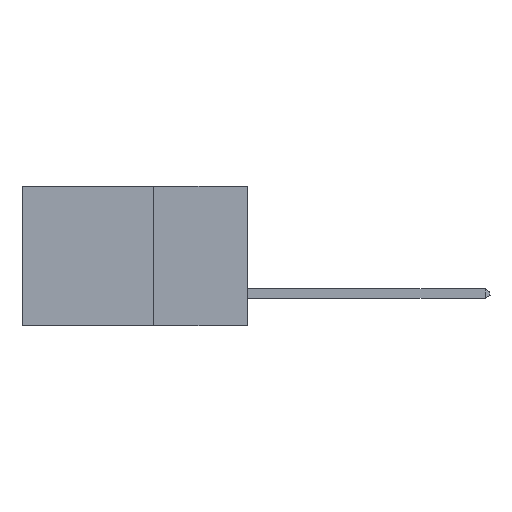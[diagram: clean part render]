
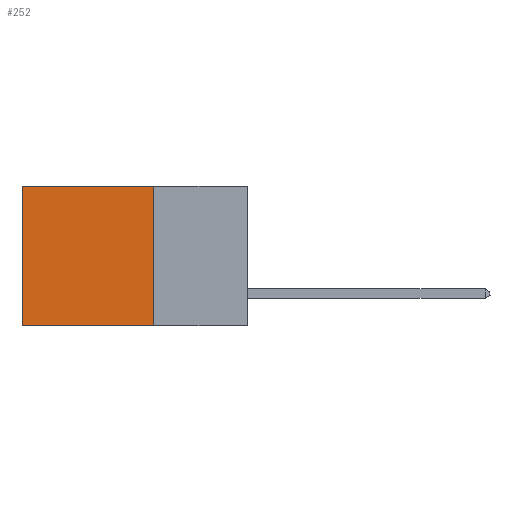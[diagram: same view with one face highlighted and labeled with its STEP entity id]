
A CAD part, left-side view. The second image highlights one B-rep face of the part: STEP entity #252.
In plain terms, the highlighted planar face has unit normal (-1, 0, 0).
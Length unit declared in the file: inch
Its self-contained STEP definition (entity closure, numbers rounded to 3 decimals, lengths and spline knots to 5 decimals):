
#252 = ADVANCED_FACE ( 'NONE', ( #9897 ), #10435, .F. ) ;
#400 = DIRECTION ( 'NONE',  ( 0., 1., 0. ) ) ;
#653 = VECTOR ( 'NONE', #4759, 39.37008 ) ;
#1250 = CARTESIAN_POINT ( 'NONE',  ( 0.298, 0.6, 0. ) ) ;
#1573 = CARTESIAN_POINT ( 'NONE',  ( 0.298, 0.6, 0. ) ) ;
#1584 = LINE ( 'NONE', #4831, #7233 ) ;
#1799 = DIRECTION ( 'NONE',  ( 0., 1., 0. ) ) ;
#3656 = CARTESIAN_POINT ( 'NONE',  ( 0.298, 0.25, 0. ) ) ;
#3745 = VERTEX_POINT ( 'NONE', #3656 ) ;
#3851 = EDGE_CURVE ( 'NONE', #3745, #8096, #1584, .T. ) ;
#4073 = LINE ( 'NONE', #1573, #653 ) ;
#4759 = DIRECTION ( 'NONE',  ( 0., 0., -1. ) ) ;
#4831 = CARTESIAN_POINT ( 'NONE',  ( 0.298, 0.25, 0. ) ) ;
#4998 = DIRECTION ( 'NONE',  ( 1., 0., 0. ) ) ;
#5397 = EDGE_CURVE ( 'NONE', #8096, #11204, #5436, .T. ) ;
#5436 = LINE ( 'NONE', #11638, #5963 ) ;
#5452 = CARTESIAN_POINT ( 'NONE',  ( 0.298, 0.25, -0.37 ) ) ;
#5945 = DIRECTION ( 'NONE',  ( 0., 0., -1. ) ) ;
#5963 = VECTOR ( 'NONE', #400, 39.37008 ) ;
#6391 = ORIENTED_EDGE ( 'NONE', *, *, #3851, .F. ) ;
#6437 = VECTOR ( 'NONE', #1799, 39.37008 ) ;
#6791 = LINE ( 'NONE', #7823, #6437 ) ;
#7233 = VECTOR ( 'NONE', #12708, 39.37008 ) ;
#7242 = ORIENTED_EDGE ( 'NONE', *, *, #8331, .T. ) ;
#7823 = CARTESIAN_POINT ( 'NONE',  ( 0.298, 0.25, 0. ) ) ;
#8096 = VERTEX_POINT ( 'NONE', #5452 ) ;
#8261 = ORIENTED_EDGE ( 'NONE', *, *, #11770, .T. ) ;
#8331 = EDGE_CURVE ( 'NONE', #11741, #11204, #4073, .T. ) ;
#8679 = EDGE_LOOP ( 'NONE', ( #7242, #14373, #6391, #8261 ) ) ;
#9400 = AXIS2_PLACEMENT_3D ( 'NONE', #12789, #4998, #5945 ) ;
#9897 = FACE_OUTER_BOUND ( 'NONE', #8679, .T. ) ;
#10435 = PLANE ( 'NONE',  #9400 ) ;
#10728 = CARTESIAN_POINT ( 'NONE',  ( 0.298, 0.6, -0.37 ) ) ;
#11204 = VERTEX_POINT ( 'NONE', #10728 ) ;
#11638 = CARTESIAN_POINT ( 'NONE',  ( 0.298, 0.25, -0.37 ) ) ;
#11741 = VERTEX_POINT ( 'NONE', #1250 ) ;
#11770 = EDGE_CURVE ( 'NONE', #3745, #11741, #6791, .T. ) ;
#12708 = DIRECTION ( 'NONE',  ( 0., 0., -1. ) ) ;
#12789 = CARTESIAN_POINT ( 'NONE',  ( 0.298, 0.25, 0. ) ) ;
#14373 = ORIENTED_EDGE ( 'NONE', *, *, #5397, .F. ) ;
